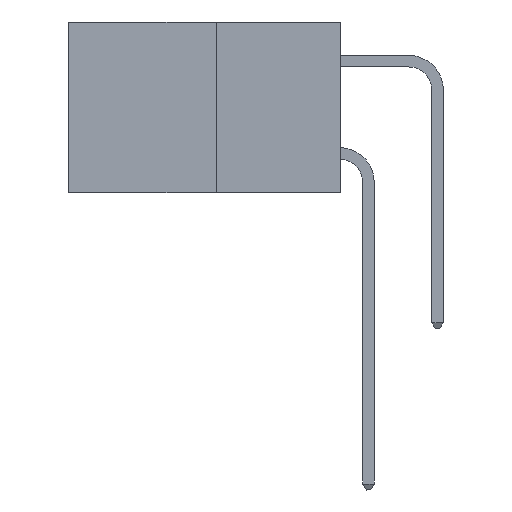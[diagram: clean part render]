
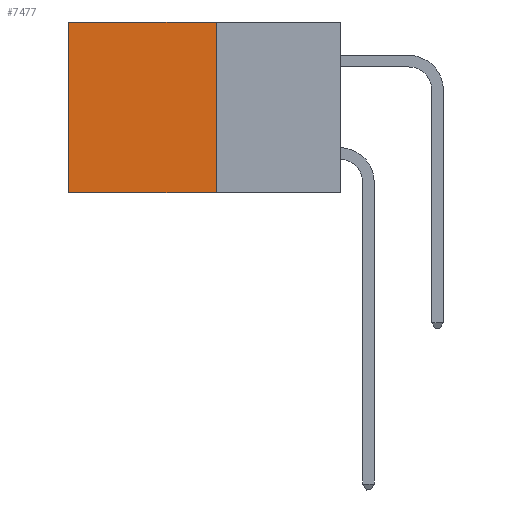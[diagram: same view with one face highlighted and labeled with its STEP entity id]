
A CAD part, left-side view. The second image highlights one B-rep face of the part: STEP entity #7477.
In plain terms, the highlighted planar face has unit normal (-1, 0, 0).
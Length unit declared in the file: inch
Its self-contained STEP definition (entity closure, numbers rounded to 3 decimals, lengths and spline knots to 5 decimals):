
#413 = ORIENTED_EDGE ( 'NONE', *, *, #8442, .T. ) ;
#962 = VECTOR ( 'NONE', #28149, 39.37008 ) ;
#2221 = CARTESIAN_POINT ( 'NONE',  ( 0.277, 0.27, 0. ) ) ;
#2447 = CARTESIAN_POINT ( 'NONE',  ( 0.277, 0.27, -0.37 ) ) ;
#7477 = ADVANCED_FACE ( 'NONE', ( #25349 ), #31464, .F. ) ;
#7950 = ORIENTED_EDGE ( 'NONE', *, *, #26724, .T. ) ;
#8442 = EDGE_CURVE ( 'NONE', #11926, #23964, #28917, .T. ) ;
#10162 = VECTOR ( 'NONE', #18769, 39.37008 ) ;
#10490 = DIRECTION ( 'NONE',  ( 0., 0., -1. ) ) ;
#10616 = CARTESIAN_POINT ( 'NONE',  ( 0.277, 0.59, -0.37 ) ) ;
#11926 = VERTEX_POINT ( 'NONE', #21743 ) ;
#12283 = CARTESIAN_POINT ( 'NONE',  ( 0.277, 0.27, 0. ) ) ;
#12631 = CARTESIAN_POINT ( 'NONE',  ( 0.277, 0.27, -0.37 ) ) ;
#15531 = LINE ( 'NONE', #12283, #962 ) ;
#16825 = VERTEX_POINT ( 'NONE', #2221 ) ;
#17857 = VECTOR ( 'NONE', #33233, 39.37008 ) ;
#18557 = EDGE_CURVE ( 'NONE', #22699, #23964, #24749, .T. ) ;
#18769 = DIRECTION ( 'NONE',  ( 0., 0., -1. ) ) ;
#19378 = EDGE_CURVE ( 'NONE', #16825, #22699, #24304, .T. ) ;
#21090 = AXIS2_PLACEMENT_3D ( 'NONE', #31817, #31389, #31380 ) ;
#21743 = CARTESIAN_POINT ( 'NONE',  ( 0.277, 0.59, 0. ) ) ;
#21984 = VECTOR ( 'NONE', #10490, 39.37008 ) ;
#22699 = VERTEX_POINT ( 'NONE', #12631 ) ;
#23964 = VERTEX_POINT ( 'NONE', #30427 ) ;
#24304 = LINE ( 'NONE', #2447, #10162 ) ;
#24749 = LINE ( 'NONE', #25439, #17857 ) ;
#25349 = FACE_OUTER_BOUND ( 'NONE', #32892, .T. ) ;
#25439 = CARTESIAN_POINT ( 'NONE',  ( 0.277, 0.27, -0.37 ) ) ;
#26717 = ORIENTED_EDGE ( 'NONE', *, *, #19378, .F. ) ;
#26724 = EDGE_CURVE ( 'NONE', #16825, #11926, #15531, .T. ) ;
#27956 = ORIENTED_EDGE ( 'NONE', *, *, #18557, .F. ) ;
#28149 = DIRECTION ( 'NONE',  ( 0., 1., 0. ) ) ;
#28917 = LINE ( 'NONE', #10616, #21984 ) ;
#30427 = CARTESIAN_POINT ( 'NONE',  ( 0.277, 0.59, -0.37 ) ) ;
#31380 = DIRECTION ( 'NONE',  ( 0., 0., -1. ) ) ;
#31389 = DIRECTION ( 'NONE',  ( 1., 0., 0. ) ) ;
#31464 = PLANE ( 'NONE',  #21090 ) ;
#31817 = CARTESIAN_POINT ( 'NONE',  ( 0.277, 0.27, -0.37 ) ) ;
#32892 = EDGE_LOOP ( 'NONE', ( #413, #27956, #26717, #7950 ) ) ;
#33233 = DIRECTION ( 'NONE',  ( 0., 1., 0. ) ) ;
